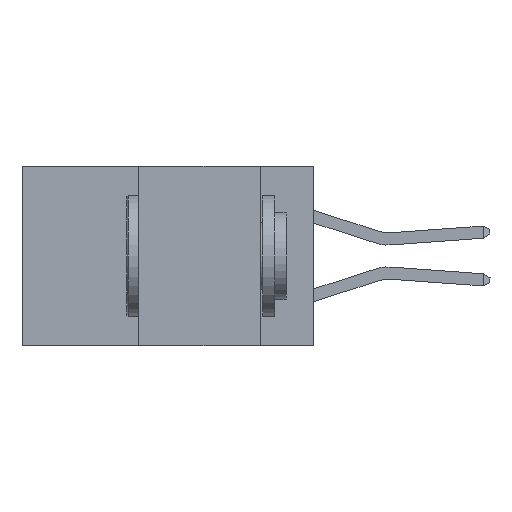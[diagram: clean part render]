
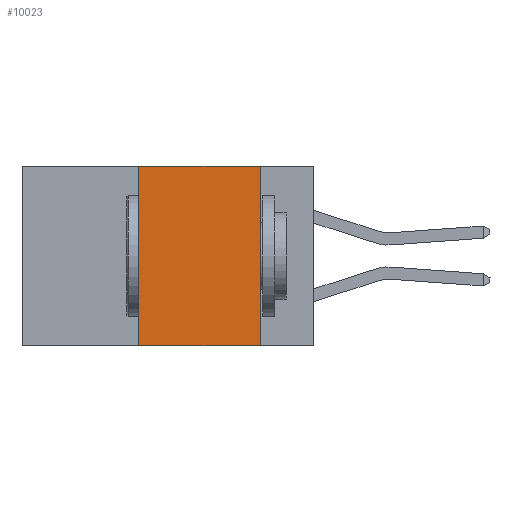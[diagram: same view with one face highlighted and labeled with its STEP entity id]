
A CAD part, left-side view. The second image highlights one B-rep face of the part: STEP entity #10023.
In plain terms, the highlighted planar face has unit normal (-1, 0, 0).
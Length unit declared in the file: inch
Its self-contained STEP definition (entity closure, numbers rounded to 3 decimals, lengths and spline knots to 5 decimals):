
#322 = DIRECTION ( 'NONE',  ( 1., 0., 0. ) ) ;
#506 = DIRECTION ( 'NONE',  ( 0., 0., 1. ) ) ;
#1404 = CARTESIAN_POINT ( 'NONE',  ( 0., 0.6, 0. ) ) ;
#1545 = CARTESIAN_POINT ( 'NONE',  ( 0., 0.36, 0. ) ) ;
#1626 = EDGE_CURVE ( 'NONE', #11406, #5106, #5906, .T. ) ;
#2842 = VECTOR ( 'NONE', #8878, 39.37008 ) ;
#2912 = VECTOR ( 'NONE', #13465, 39.37008 ) ;
#3265 = FACE_OUTER_BOUND ( 'NONE', #5643, .T. ) ;
#4055 = LINE ( 'NONE', #1545, #10236 ) ;
#4659 = CARTESIAN_POINT ( 'NONE',  ( 0., 0.11, -0.37 ) ) ;
#5074 = LINE ( 'NONE', #12341, #2912 ) ;
#5106 = VERTEX_POINT ( 'NONE', #14346 ) ;
#5643 = EDGE_LOOP ( 'NONE', ( #14989, #12761, #12634, #7529 ) ) ;
#5906 = LINE ( 'NONE', #6461, #2842 ) ;
#5997 = AXIS2_PLACEMENT_3D ( 'NONE', #1404, #322, #6078 ) ;
#6078 = DIRECTION ( 'NONE',  ( 0., 0., -1. ) ) ;
#6461 = CARTESIAN_POINT ( 'NONE',  ( 0., 0.6, 0. ) ) ;
#6510 = EDGE_CURVE ( 'NONE', #8751, #11406, #4055, .T. ) ;
#7529 = ORIENTED_EDGE ( 'NONE', *, *, #8534, .T. ) ;
#8333 = VECTOR ( 'NONE', #11102, 39.37008 ) ;
#8454 = EDGE_CURVE ( 'NONE', #5106, #10938, #8711, .T. ) ;
#8534 = EDGE_CURVE ( 'NONE', #8751, #10938, #5074, .T. ) ;
#8711 = LINE ( 'NONE', #14531, #8333 ) ;
#8751 = VERTEX_POINT ( 'NONE', #9052 ) ;
#8878 = DIRECTION ( 'NONE',  ( 0., -1., 0. ) ) ;
#9052 = CARTESIAN_POINT ( 'NONE',  ( 0., 0.36, -0.37 ) ) ;
#10023 = ADVANCED_FACE ( 'NONE', ( #3265 ), #12923, .F. ) ;
#10236 = VECTOR ( 'NONE', #506, 39.37008 ) ;
#10616 = CARTESIAN_POINT ( 'NONE',  ( 0., 0.36, 0. ) ) ;
#10938 = VERTEX_POINT ( 'NONE', #4659 ) ;
#11102 = DIRECTION ( 'NONE',  ( 0., 0., -1. ) ) ;
#11406 = VERTEX_POINT ( 'NONE', #10616 ) ;
#12341 = CARTESIAN_POINT ( 'NONE',  ( 0., 0.6, -0.37 ) ) ;
#12634 = ORIENTED_EDGE ( 'NONE', *, *, #6510, .F. ) ;
#12761 = ORIENTED_EDGE ( 'NONE', *, *, #1626, .F. ) ;
#12923 = PLANE ( 'NONE',  #5997 ) ;
#13465 = DIRECTION ( 'NONE',  ( 0., -1., 0. ) ) ;
#14346 = CARTESIAN_POINT ( 'NONE',  ( 0., 0.11, 0. ) ) ;
#14531 = CARTESIAN_POINT ( 'NONE',  ( 0., 0.11, 0. ) ) ;
#14989 = ORIENTED_EDGE ( 'NONE', *, *, #8454, .F. ) ;
